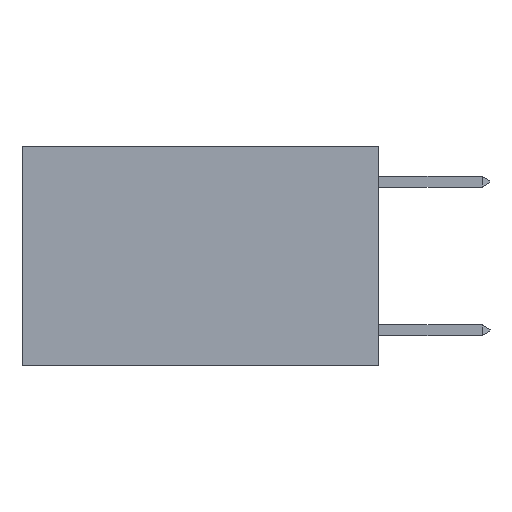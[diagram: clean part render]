
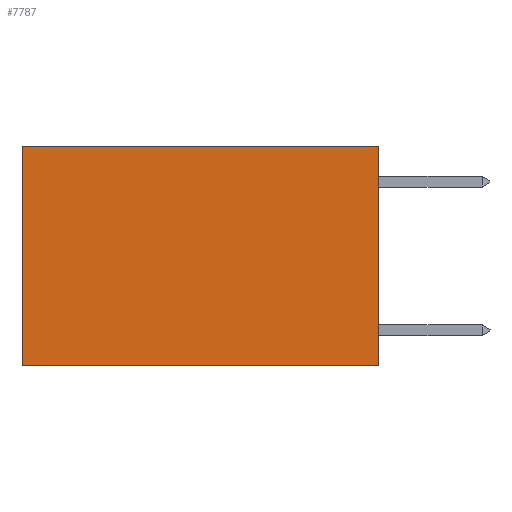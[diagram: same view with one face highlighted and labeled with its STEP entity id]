
A CAD part, left-side view. The second image highlights one B-rep face of the part: STEP entity #7787.
In plain terms, the highlighted planar face has unit normal (-1, 0, 0).
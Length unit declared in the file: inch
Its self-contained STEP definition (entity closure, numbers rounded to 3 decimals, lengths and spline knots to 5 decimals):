
#2210 = VECTOR ( 'NONE', #22219, 39.37008 ) ;
#2800 = CARTESIAN_POINT ( 'NONE',  ( 0.2625, 0., 0. ) ) ;
#3296 = CARTESIAN_POINT ( 'NONE',  ( 0.2625, 0.6, -0.37 ) ) ;
#3412 = DIRECTION ( 'NONE',  ( 0., 1., 0. ) ) ;
#3930 = EDGE_CURVE ( 'NONE', #13594, #16186, #23953, .T. ) ;
#3946 = ORIENTED_EDGE ( 'NONE', *, *, #11579, .F. ) ;
#4442 = CARTESIAN_POINT ( 'NONE',  ( 0.2625, 0., -0.37 ) ) ;
#5849 = CARTESIAN_POINT ( 'NONE',  ( 0.2625, 0., 0. ) ) ;
#6179 = FACE_OUTER_BOUND ( 'NONE', #31126, .T. ) ;
#6738 = EDGE_CURVE ( 'NONE', #19062, #13594, #10801, .T. ) ;
#7621 = CARTESIAN_POINT ( 'NONE',  ( 0.2625, 0., 0. ) ) ;
#7787 = ADVANCED_FACE ( 'NONE', ( #6179 ), #19636, .F. ) ;
#8506 = ORIENTED_EDGE ( 'NONE', *, *, #3930, .T. ) ;
#8667 = LINE ( 'NONE', #2800, #2210 ) ;
#8951 = ORIENTED_EDGE ( 'NONE', *, *, #28293, .F. ) ;
#9063 = CARTESIAN_POINT ( 'NONE',  ( 0.2625, 0., -0.37 ) ) ;
#10063 = DIRECTION ( 'NONE',  ( 0., 0., -1. ) ) ;
#10801 = LINE ( 'NONE', #5849, #22947 ) ;
#11579 = EDGE_CURVE ( 'NONE', #18395, #16186, #24857, .T. ) ;
#13594 = VERTEX_POINT ( 'NONE', #30483 ) ;
#15155 = ORIENTED_EDGE ( 'NONE', *, *, #6738, .T. ) ;
#16186 = VERTEX_POINT ( 'NONE', #3296 ) ;
#17498 = VECTOR ( 'NONE', #31354, 39.37008 ) ;
#18395 = VERTEX_POINT ( 'NONE', #9063 ) ;
#19062 = VERTEX_POINT ( 'NONE', #27431 ) ;
#19583 = AXIS2_PLACEMENT_3D ( 'NONE', #7621, #24587, #10063 ) ;
#19636 = PLANE ( 'NONE',  #19583 ) ;
#22219 = DIRECTION ( 'NONE',  ( 0., 0., -1. ) ) ;
#22947 = VECTOR ( 'NONE', #3412, 39.37008 ) ;
#23953 = LINE ( 'NONE', #31246, #17498 ) ;
#24097 = VECTOR ( 'NONE', #28692, 39.37008 ) ;
#24587 = DIRECTION ( 'NONE',  ( 1., 0., 0. ) ) ;
#24857 = LINE ( 'NONE', #4442, #24097 ) ;
#27431 = CARTESIAN_POINT ( 'NONE',  ( 0.2625, 0., 0. ) ) ;
#28293 = EDGE_CURVE ( 'NONE', #19062, #18395, #8667, .T. ) ;
#28692 = DIRECTION ( 'NONE',  ( 0., 1., 0. ) ) ;
#30483 = CARTESIAN_POINT ( 'NONE',  ( 0.2625, 0.6, 0. ) ) ;
#31126 = EDGE_LOOP ( 'NONE', ( #8506, #3946, #8951, #15155 ) ) ;
#31246 = CARTESIAN_POINT ( 'NONE',  ( 0.2625, 0.6, 0. ) ) ;
#31354 = DIRECTION ( 'NONE',  ( 0., 0., -1. ) ) ;
